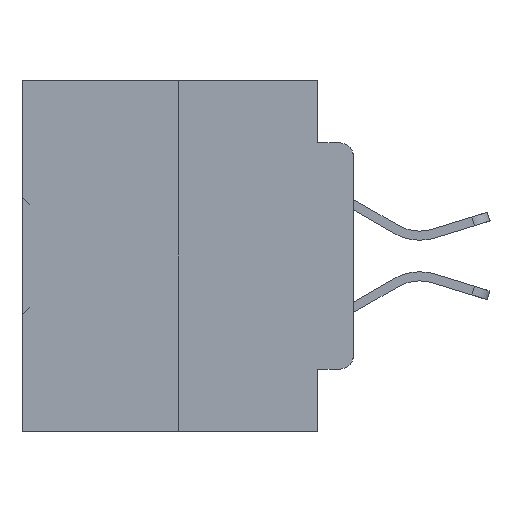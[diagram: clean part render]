
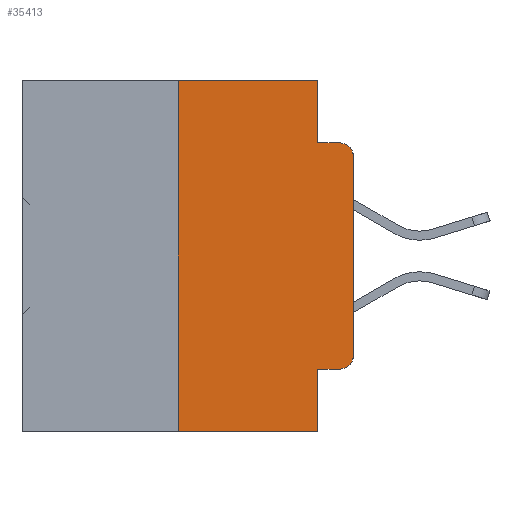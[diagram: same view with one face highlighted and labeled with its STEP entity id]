
A CAD part, left-side view. The second image highlights one B-rep face of the part: STEP entity #35413.
In plain terms, the highlighted planar face has unit normal (-1, 0, 0).
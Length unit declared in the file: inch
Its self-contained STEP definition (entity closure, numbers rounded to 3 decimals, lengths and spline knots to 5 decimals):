
#112 = CARTESIAN_POINT ( 'NONE',  ( 0., 0.051, -0.4115 ) ) ;
#433 = CARTESIAN_POINT ( 'NONE',  ( 0., 0., -0.3915 ) ) ;
#1114 = CARTESIAN_POINT ( 'NONE',  ( 0., 0.473, 0. ) ) ;
#1223 = VERTEX_POINT ( 'NONE', #9188 ) ;
#2104 = VECTOR ( 'NONE', #31547, 39.37008 ) ;
#2242 = ORIENTED_EDGE ( 'NONE', *, *, #34091, .F. ) ;
#2828 = LINE ( 'NONE', #23749, #10596 ) ;
#3654 = LINE ( 'NONE', #27704, #23311 ) ;
#4012 = CARTESIAN_POINT ( 'NONE',  ( 0., 0., -0.1085 ) ) ;
#4321 = CARTESIAN_POINT ( 'NONE',  ( 0., 0.051, 0. ) ) ;
#5361 = EDGE_CURVE ( 'NONE', #11542, #26453, #2828, .T. ) ;
#6834 = LINE ( 'NONE', #18763, #19512 ) ;
#7378 = EDGE_CURVE ( 'NONE', #31063, #26218, #22727, .T. ) ;
#7508 = ORIENTED_EDGE ( 'NONE', *, *, #10599, .T. ) ;
#8536 = VERTEX_POINT ( 'NONE', #30836 ) ;
#9188 = CARTESIAN_POINT ( 'NONE',  ( 0., 0.02, -0.4115 ) ) ;
#9241 = VERTEX_POINT ( 'NONE', #28414 ) ;
#10232 = AXIS2_PLACEMENT_3D ( 'NONE', #1114, #36217, #24270 ) ;
#10331 = CARTESIAN_POINT ( 'NONE',  ( 0., 0.051, -0.5 ) ) ;
#10596 = VECTOR ( 'NONE', #20431, 39.37008 ) ;
#10599 = EDGE_CURVE ( 'NONE', #8536, #26453, #11012, .T. ) ;
#11012 = LINE ( 'NONE', #22969, #17332 ) ;
#11014 = ORIENTED_EDGE ( 'NONE', *, *, #24288, .F. ) ;
#11049 = CARTESIAN_POINT ( 'NONE',  ( 0., 0.02, -0.1085 ) ) ;
#11542 = VERTEX_POINT ( 'NONE', #112 ) ;
#12693 = EDGE_CURVE ( 'NONE', #1223, #30366, #32910, .T. ) ;
#13243 = PLANE ( 'NONE',  #10232 ) ;
#13269 = VERTEX_POINT ( 'NONE', #23976 ) ;
#13989 = DIRECTION ( 'NONE',  ( 0., 0., -1. ) ) ;
#14130 = DIRECTION ( 'NONE',  ( 0., -1., 0. ) ) ;
#14175 = DIRECTION ( 'NONE',  ( -1., 0., 0. ) ) ;
#14411 = VECTOR ( 'NONE', #16449, 39.37008 ) ;
#15947 = AXIS2_PLACEMENT_3D ( 'NONE', #11049, #14175, #13989 ) ;
#16449 = DIRECTION ( 'NONE',  ( 0., 0., -1. ) ) ;
#16652 = LINE ( 'NONE', #19785, #2104 ) ;
#17281 = AXIS2_PLACEMENT_3D ( 'NONE', #20117, #22669, #25972 ) ;
#17332 = VECTOR ( 'NONE', #14130, 39.37008 ) ;
#17521 = EDGE_CURVE ( 'NONE', #11542, #1223, #23486, .T. ) ;
#18035 = ORIENTED_EDGE ( 'NONE', *, *, #36915, .T. ) ;
#18630 = LINE ( 'NONE', #36636, #34043 ) ;
#18763 = CARTESIAN_POINT ( 'NONE',  ( 0., 0., 0. ) ) ;
#19512 = VECTOR ( 'NONE', #30699, 39.37008 ) ;
#19785 = CARTESIAN_POINT ( 'NONE',  ( 0., 0.25, 0. ) ) ;
#20117 = CARTESIAN_POINT ( 'NONE',  ( 0., 0.02, -0.3915 ) ) ;
#20431 = DIRECTION ( 'NONE',  ( 0., 0., -1. ) ) ;
#20877 = VERTEX_POINT ( 'NONE', #4012 ) ;
#21022 = ORIENTED_EDGE ( 'NONE', *, *, #7378, .F. ) ;
#22164 = ORIENTED_EDGE ( 'NONE', *, *, #5361, .F. ) ;
#22669 = DIRECTION ( 'NONE',  ( -1., 0., 0. ) ) ;
#22727 = LINE ( 'NONE', #4321, #14411 ) ;
#22969 = CARTESIAN_POINT ( 'NONE',  ( 0., 0.473, -0.5 ) ) ;
#23311 = VECTOR ( 'NONE', #30645, 39.37008 ) ;
#23486 = LINE ( 'NONE', #38539, #36169 ) ;
#23749 = CARTESIAN_POINT ( 'NONE',  ( 0., 0.051, 0. ) ) ;
#23976 = CARTESIAN_POINT ( 'NONE',  ( 0., 0.25, 0. ) ) ;
#24270 = DIRECTION ( 'NONE',  ( 0., 0., -1. ) ) ;
#24288 = EDGE_CURVE ( 'NONE', #8536, #13269, #16652, .T. ) ;
#25957 = CIRCLE ( 'NONE', #15947, 0.02 ) ;
#25972 = DIRECTION ( 'NONE',  ( 0., 0., -1. ) ) ;
#26009 = CARTESIAN_POINT ( 'NONE',  ( 0., 0.051, -0.0885 ) ) ;
#26218 = VERTEX_POINT ( 'NONE', #26009 ) ;
#26453 = VERTEX_POINT ( 'NONE', #10331 ) ;
#26996 = ORIENTED_EDGE ( 'NONE', *, *, #17521, .T. ) ;
#27704 = CARTESIAN_POINT ( 'NONE',  ( 0., 0.473, 0. ) ) ;
#28414 = CARTESIAN_POINT ( 'NONE',  ( 0., 0.02, -0.0885 ) ) ;
#28902 = CARTESIAN_POINT ( 'NONE',  ( 0., 0.051, 0. ) ) ;
#30134 = FACE_OUTER_BOUND ( 'NONE', #32235, .T. ) ;
#30366 = VERTEX_POINT ( 'NONE', #433 ) ;
#30378 = DIRECTION ( 'NONE',  ( 0., -1., 0. ) ) ;
#30645 = DIRECTION ( 'NONE',  ( 0., -1., 0. ) ) ;
#30699 = DIRECTION ( 'NONE',  ( 0., 0., 1. ) ) ;
#30735 = ORIENTED_EDGE ( 'NONE', *, *, #33771, .T. ) ;
#30836 = CARTESIAN_POINT ( 'NONE',  ( 0., 0.25, -0.5 ) ) ;
#31063 = VERTEX_POINT ( 'NONE', #28902 ) ;
#31547 = DIRECTION ( 'NONE',  ( 0., 0., 1. ) ) ;
#32235 = EDGE_LOOP ( 'NONE', ( #30735, #18035, #34069, #21022, #2242, #11014, #7508, #22164, #26996, #33916 ) ) ;
#32482 = DIRECTION ( 'NONE',  ( 0., -1., 0. ) ) ;
#32910 = CIRCLE ( 'NONE', #17281, 0.02 ) ;
#33771 = EDGE_CURVE ( 'NONE', #30366, #20877, #6834, .T. ) ;
#33916 = ORIENTED_EDGE ( 'NONE', *, *, #12693, .T. ) ;
#34043 = VECTOR ( 'NONE', #30378, 39.37008 ) ;
#34069 = ORIENTED_EDGE ( 'NONE', *, *, #36310, .F. ) ;
#34091 = EDGE_CURVE ( 'NONE', #13269, #31063, #3654, .T. ) ;
#35413 = ADVANCED_FACE ( 'NONE', ( #30134 ), #13243, .F. ) ;
#36169 = VECTOR ( 'NONE', #32482, 39.37008 ) ;
#36217 = DIRECTION ( 'NONE',  ( 1., 0., 0. ) ) ;
#36310 = EDGE_CURVE ( 'NONE', #26218, #9241, #18630, .T. ) ;
#36636 = CARTESIAN_POINT ( 'NONE',  ( 0., 0.051, -0.0885 ) ) ;
#36915 = EDGE_CURVE ( 'NONE', #20877, #9241, #25957, .T. ) ;
#38539 = CARTESIAN_POINT ( 'NONE',  ( 0., 0.051, -0.4115 ) ) ;
